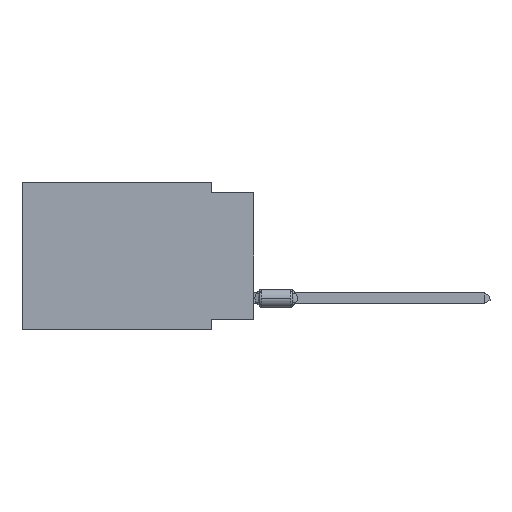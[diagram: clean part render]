
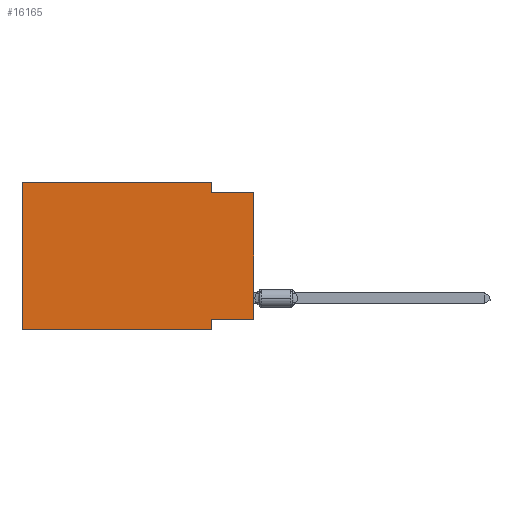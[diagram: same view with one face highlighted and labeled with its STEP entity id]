
A CAD part, left-side view. The second image highlights one B-rep face of the part: STEP entity #16165.
In plain terms, the highlighted planar face has unit normal (-1, 0, 0).
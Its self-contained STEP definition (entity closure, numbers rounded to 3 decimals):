
#149 = DIRECTION ( 'NONE',  ( 1., 0., 0. ) ) ;
#188 = EDGE_CURVE ( 'NONE', #3291, #17676, #1466, .T. ) ;
#532 = AXIS2_PLACEMENT_3D ( 'NONE', #12666, #149, #5718 ) ;
#1440 = FACE_OUTER_BOUND ( 'NONE', #7045, .T. ) ;
#1466 = LINE ( 'NONE', #5654, #14312 ) ;
#2953 = CARTESIAN_POINT ( 'NONE',  ( 0., 13.97, -8.89 ) ) ;
#3240 = CARTESIAN_POINT ( 'NONE',  ( 0., 13.97, 0. ) ) ;
#3252 = EDGE_CURVE ( 'NONE', #13273, #3291, #12608, .T. ) ;
#3287 = VECTOR ( 'NONE', #11982, 1000. ) ;
#3291 = VERTEX_POINT ( 'NONE', #16041 ) ;
#3876 = EDGE_CURVE ( 'NONE', #7329, #6040, #4964, .T. ) ;
#4093 = EDGE_CURVE ( 'NONE', #17676, #6162, #13196, .T. ) ;
#4964 = LINE ( 'NONE', #13460, #3287 ) ;
#5461 = ORIENTED_EDGE ( 'NONE', *, *, #12275, .F. ) ;
#5654 = CARTESIAN_POINT ( 'NONE',  ( 0., 2.54, 0. ) ) ;
#5718 = DIRECTION ( 'NONE',  ( 0., 0., -1. ) ) ;
#5762 = ORIENTED_EDGE ( 'NONE', *, *, #4093, .F. ) ;
#5988 = DIRECTION ( 'NONE',  ( 0., -1., 0. ) ) ;
#6040 = VERTEX_POINT ( 'NONE', #15739 ) ;
#6162 = VERTEX_POINT ( 'NONE', #9223 ) ;
#6364 = DIRECTION ( 'NONE',  ( 0., 0., 1. ) ) ;
#6905 = CARTESIAN_POINT ( 'NONE',  ( 0., 0., -8.255 ) ) ;
#7045 = EDGE_LOOP ( 'NONE', ( #8689, #5762, #15881, #15825, #5461, #10144, #12688, #16689 ) ) ;
#7094 = PLANE ( 'NONE',  #532 ) ;
#7216 = DIRECTION ( 'NONE',  ( 0., 1., 0. ) ) ;
#7329 = VERTEX_POINT ( 'NONE', #14326 ) ;
#7430 = DIRECTION ( 'NONE',  ( 0., 0., 1. ) ) ;
#7479 = LINE ( 'NONE', #8502, #9578 ) ;
#8000 = VECTOR ( 'NONE', #17399, 1000. ) ;
#8502 = CARTESIAN_POINT ( 'NONE',  ( 0., 0., -8.255 ) ) ;
#8689 = ORIENTED_EDGE ( 'NONE', *, *, #10642, .T. ) ;
#8929 = CARTESIAN_POINT ( 'NONE',  ( 0., 0., 0. ) ) ;
#9223 = CARTESIAN_POINT ( 'NONE',  ( 0., 0., -0.635 ) ) ;
#9356 = VERTEX_POINT ( 'NONE', #2953 ) ;
#9578 = VECTOR ( 'NONE', #7216, 1000. ) ;
#9703 = EDGE_CURVE ( 'NONE', #17567, #7329, #7479, .T. ) ;
#10091 = CARTESIAN_POINT ( 'NONE',  ( 0., 2.54, -0.635 ) ) ;
#10144 = ORIENTED_EDGE ( 'NONE', *, *, #17435, .T. ) ;
#10256 = CARTESIAN_POINT ( 'NONE',  ( 0., 13.97, 0. ) ) ;
#10392 = LINE ( 'NONE', #8929, #15468 ) ;
#10642 = EDGE_CURVE ( 'NONE', #17567, #6162, #10392, .T. ) ;
#10745 = CARTESIAN_POINT ( 'NONE',  ( 0., 13.97, -8.89 ) ) ;
#10965 = VECTOR ( 'NONE', #7430, 1000. ) ;
#11228 = DIRECTION ( 'NONE',  ( 0., 0., -1. ) ) ;
#11819 = CARTESIAN_POINT ( 'NONE',  ( 0., 0., -0.635 ) ) ;
#11884 = CARTESIAN_POINT ( 'NONE',  ( 0., 13.97, 0. ) ) ;
#11982 = DIRECTION ( 'NONE',  ( 0., 0., -1. ) ) ;
#12275 = EDGE_CURVE ( 'NONE', #9356, #13273, #13359, .T. ) ;
#12608 = LINE ( 'NONE', #3240, #17025 ) ;
#12666 = CARTESIAN_POINT ( 'NONE',  ( 0., 13.97, 0. ) ) ;
#12688 = ORIENTED_EDGE ( 'NONE', *, *, #3876, .F. ) ;
#13196 = LINE ( 'NONE', #11819, #8000 ) ;
#13273 = VERTEX_POINT ( 'NONE', #11884 ) ;
#13359 = LINE ( 'NONE', #10256, #10965 ) ;
#13398 = DIRECTION ( 'NONE',  ( 0., -1., 0. ) ) ;
#13428 = VECTOR ( 'NONE', #13398, 1000. ) ;
#13460 = CARTESIAN_POINT ( 'NONE',  ( 0., 2.54, -8.89 ) ) ;
#14312 = VECTOR ( 'NONE', #11228, 1000. ) ;
#14326 = CARTESIAN_POINT ( 'NONE',  ( 0., 2.54, -8.255 ) ) ;
#15468 = VECTOR ( 'NONE', #6364, 1000. ) ;
#15739 = CARTESIAN_POINT ( 'NONE',  ( 0., 2.54, -8.89 ) ) ;
#15825 = ORIENTED_EDGE ( 'NONE', *, *, #3252, .F. ) ;
#15881 = ORIENTED_EDGE ( 'NONE', *, *, #188, .F. ) ;
#16041 = CARTESIAN_POINT ( 'NONE',  ( 0., 2.54, 0. ) ) ;
#16165 = ADVANCED_FACE ( 'NONE', ( #1440 ), #7094, .F. ) ;
#16689 = ORIENTED_EDGE ( 'NONE', *, *, #9703, .F. ) ;
#16989 = LINE ( 'NONE', #10745, #13428 ) ;
#17025 = VECTOR ( 'NONE', #5988, 1000. ) ;
#17399 = DIRECTION ( 'NONE',  ( 0., -1., 0. ) ) ;
#17435 = EDGE_CURVE ( 'NONE', #9356, #6040, #16989, .T. ) ;
#17567 = VERTEX_POINT ( 'NONE', #6905 ) ;
#17676 = VERTEX_POINT ( 'NONE', #10091 ) ;
